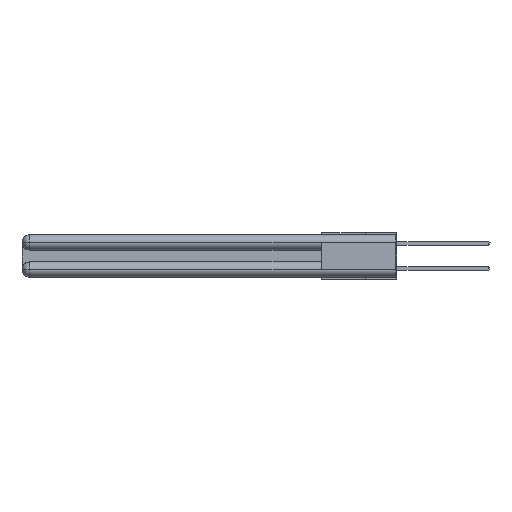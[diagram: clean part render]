
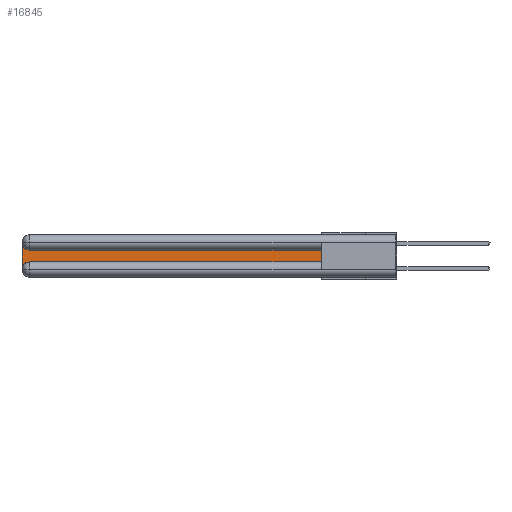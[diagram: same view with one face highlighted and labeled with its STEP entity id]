
A CAD part, left-side view. The second image highlights one B-rep face of the part: STEP entity #16845.
In plain terms, the highlighted planar face has unit normal (-1, 0, 0).
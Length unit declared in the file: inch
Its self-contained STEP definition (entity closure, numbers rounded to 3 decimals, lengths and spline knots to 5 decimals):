
#931 = ORIENTED_EDGE ( 'NONE', *, *, #30376, .T. ) ;
#1041 = CARTESIAN_POINT ( 'NONE',  ( 0.075, 3., -0.2175 ) ) ;
#2388 = AXIS2_PLACEMENT_3D ( 'NONE', #19474, #3902, #16557 ) ;
#2613 = VERTEX_POINT ( 'NONE', #12779 ) ;
#3071 = EDGE_LOOP ( 'NONE', ( #21686, #931, #30807, #26548, #3859, #30958 ) ) ;
#3289 = VERTEX_POINT ( 'NONE', #7351 ) ;
#3442 = VECTOR ( 'NONE', #3642, 39.37008 ) ;
#3642 = DIRECTION ( 'NONE',  ( 0., 0., -1. ) ) ;
#3660 = DIRECTION ( 'NONE',  ( 0., 0., 1. ) ) ;
#3859 = ORIENTED_EDGE ( 'NONE', *, *, #6184, .T. ) ;
#3902 = DIRECTION ( 'NONE',  ( 1., 0., 0. ) ) ;
#5577 = CIRCLE ( 'NONE', #23177, 0.06 ) ;
#6184 = EDGE_CURVE ( 'NONE', #3289, #22328, #14579, .T. ) ;
#6978 = EDGE_CURVE ( 'NONE', #31076, #3289, #5577, .T. ) ;
#7351 = CARTESIAN_POINT ( 'NONE',  ( 0.075, 2.94, -0.2175 ) ) ;
#8129 = DIRECTION ( 'NONE',  ( 0., 1., 0. ) ) ;
#8555 = EDGE_CURVE ( 'NONE', #25983, #33291, #31200, .T. ) ;
#8817 = CARTESIAN_POINT ( 'NONE',  ( 0.075, 0.6, -0.2175 ) ) ;
#8966 = FACE_OUTER_BOUND ( 'NONE', #3071, .T. ) ;
#10975 = DIRECTION ( 'NONE',  ( 1., 0., 0. ) ) ;
#11138 = CIRCLE ( 'NONE', #2388, 0.06 ) ;
#12779 = CARTESIAN_POINT ( 'NONE',  ( 0.075, 3., -0.0625 ) ) ;
#12829 = VECTOR ( 'NONE', #3660, 39.37008 ) ;
#14579 = LINE ( 'NONE', #23178, #25786 ) ;
#14782 = CARTESIAN_POINT ( 'NONE',  ( 0.075, 2.94, -0.1225 ) ) ;
#15494 = CARTESIAN_POINT ( 'NONE',  ( 0.075, 3., -0.2775 ) ) ;
#16051 = AXIS2_PLACEMENT_3D ( 'NONE', #23791, #10975, #29926 ) ;
#16557 = DIRECTION ( 'NONE',  ( 0., 0., -1. ) ) ;
#16845 = ADVANCED_FACE ( 'NONE', ( #8966 ), #18635, .F. ) ;
#16909 = DIRECTION ( 'NONE',  ( 0., 0., -1. ) ) ;
#17020 = DIRECTION ( 'NONE',  ( 1., 0., 0. ) ) ;
#18131 = CARTESIAN_POINT ( 'NONE',  ( 0.075, 0.6, -0.1225 ) ) ;
#18635 = PLANE ( 'NONE',  #16051 ) ;
#19474 = CARTESIAN_POINT ( 'NONE',  ( 0.075, 2.94, -0.0625 ) ) ;
#20910 = EDGE_CURVE ( 'NONE', #2613, #31076, #30788, .T. ) ;
#21686 = ORIENTED_EDGE ( 'NONE', *, *, #8555, .T. ) ;
#22328 = VERTEX_POINT ( 'NONE', #8817 ) ;
#23177 = AXIS2_PLACEMENT_3D ( 'NONE', #27096, #17020, #16909 ) ;
#23178 = CARTESIAN_POINT ( 'NONE',  ( 0.075, 0.6, -0.2175 ) ) ;
#23293 = DIRECTION ( 'NONE',  ( 0., -1., 0. ) ) ;
#23791 = CARTESIAN_POINT ( 'NONE',  ( 0.075, 3., -0.1225 ) ) ;
#25699 = LINE ( 'NONE', #32065, #12829 ) ;
#25786 = VECTOR ( 'NONE', #23293, 39.37008 ) ;
#25887 = CARTESIAN_POINT ( 'NONE',  ( 0.075, 0.6, -0.1225 ) ) ;
#25983 = VERTEX_POINT ( 'NONE', #18131 ) ;
#26548 = ORIENTED_EDGE ( 'NONE', *, *, #6978, .T. ) ;
#27096 = CARTESIAN_POINT ( 'NONE',  ( 0.075, 2.94, -0.2775 ) ) ;
#28968 = EDGE_CURVE ( 'NONE', #22328, #25983, #25699, .T. ) ;
#29926 = DIRECTION ( 'NONE',  ( 0., 0., -1. ) ) ;
#30376 = EDGE_CURVE ( 'NONE', #33291, #2613, #11138, .T. ) ;
#30788 = LINE ( 'NONE', #1041, #3442 ) ;
#30807 = ORIENTED_EDGE ( 'NONE', *, *, #20910, .T. ) ;
#30958 = ORIENTED_EDGE ( 'NONE', *, *, #28968, .T. ) ;
#31076 = VERTEX_POINT ( 'NONE', #15494 ) ;
#31200 = LINE ( 'NONE', #25887, #31605 ) ;
#31605 = VECTOR ( 'NONE', #8129, 39.37008 ) ;
#32065 = CARTESIAN_POINT ( 'NONE',  ( 0.075, 0.6, -0.2175 ) ) ;
#33291 = VERTEX_POINT ( 'NONE', #14782 ) ;
